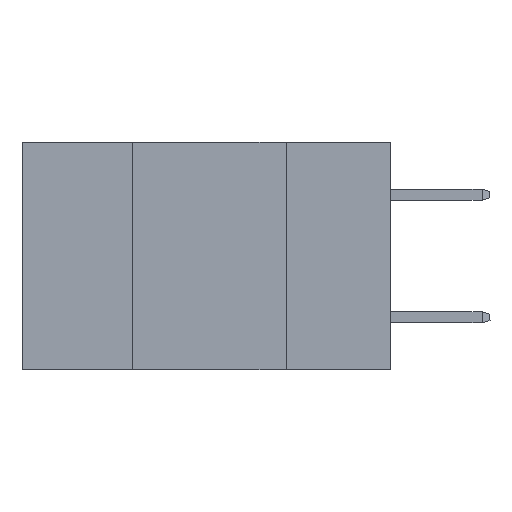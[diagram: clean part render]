
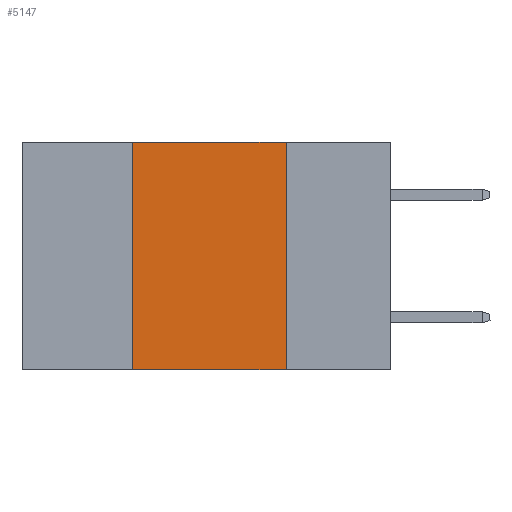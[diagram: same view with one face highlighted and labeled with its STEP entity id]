
A CAD part, left-side view. The second image highlights one B-rep face of the part: STEP entity #5147.
In plain terms, the highlighted planar face has unit normal (-1, 0, 0).
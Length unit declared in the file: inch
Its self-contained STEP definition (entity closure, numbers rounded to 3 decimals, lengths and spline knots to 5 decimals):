
#138 = CARTESIAN_POINT ( 'NONE',  ( 0., 0.17, 0. ) ) ;
#139 = CARTESIAN_POINT ( 'NONE',  ( 0., 0.17, -0.37 ) ) ;
#272 = CARTESIAN_POINT ( 'NONE',  ( 0., 0.6, -0.37 ) ) ;
#1351 = ORIENTED_EDGE ( 'NONE', *, *, #6061, .F. ) ;
#1464 = CARTESIAN_POINT ( 'NONE',  ( 0., 0.42, -0.37 ) ) ;
#1531 = ORIENTED_EDGE ( 'NONE', *, *, #8200, .F. ) ;
#2446 = VERTEX_POINT ( 'NONE', #3918 ) ;
#2653 = VECTOR ( 'NONE', #7823, 39.37008 ) ;
#2678 = CARTESIAN_POINT ( 'NONE',  ( 0., 0.6, 0. ) ) ;
#3166 = EDGE_LOOP ( 'NONE', ( #1351, #10762, #1531, #3851 ) ) ;
#3255 = EDGE_CURVE ( 'NONE', #2446, #3881, #9242, .T. ) ;
#3414 = VECTOR ( 'NONE', #8136, 39.37008 ) ;
#3851 = ORIENTED_EDGE ( 'NONE', *, *, #4118, .T. ) ;
#3881 = VERTEX_POINT ( 'NONE', #138 ) ;
#3918 = CARTESIAN_POINT ( 'NONE',  ( 0., 0.42, 0. ) ) ;
#4118 = EDGE_CURVE ( 'NONE', #8185, #5518, #8478, .T. ) ;
#4602 = LINE ( 'NONE', #7163, #2653 ) ;
#5147 = ADVANCED_FACE ( 'NONE', ( #6806 ), #6087, .F. ) ;
#5518 = VERTEX_POINT ( 'NONE', #139 ) ;
#5649 = LINE ( 'NONE', #8955, #10125 ) ;
#6061 = EDGE_CURVE ( 'NONE', #3881, #5518, #4602, .T. ) ;
#6087 = PLANE ( 'NONE',  #10504 ) ;
#6806 = FACE_OUTER_BOUND ( 'NONE', #3166, .T. ) ;
#7163 = CARTESIAN_POINT ( 'NONE',  ( 0., 0.17, 0. ) ) ;
#7520 = CARTESIAN_POINT ( 'NONE',  ( 0., 0.6, 0. ) ) ;
#7602 = DIRECTION ( 'NONE',  ( 0., -1., 0. ) ) ;
#7823 = DIRECTION ( 'NONE',  ( 0., 0., -1. ) ) ;
#8136 = DIRECTION ( 'NONE',  ( 0., -1., 0. ) ) ;
#8185 = VERTEX_POINT ( 'NONE', #1464 ) ;
#8200 = EDGE_CURVE ( 'NONE', #8185, #2446, #5649, .T. ) ;
#8478 = LINE ( 'NONE', #272, #9001 ) ;
#8508 = DIRECTION ( 'NONE',  ( 0., 0., -1. ) ) ;
#8955 = CARTESIAN_POINT ( 'NONE',  ( 0., 0.42, 0. ) ) ;
#9001 = VECTOR ( 'NONE', #7602, 39.37008 ) ;
#9242 = LINE ( 'NONE', #7520, #3414 ) ;
#9464 = DIRECTION ( 'NONE',  ( 1., 0., 0. ) ) ;
#9893 = DIRECTION ( 'NONE',  ( 0., 0., 1. ) ) ;
#10125 = VECTOR ( 'NONE', #9893, 39.37008 ) ;
#10504 = AXIS2_PLACEMENT_3D ( 'NONE', #2678, #9464, #8508 ) ;
#10762 = ORIENTED_EDGE ( 'NONE', *, *, #3255, .F. ) ;
